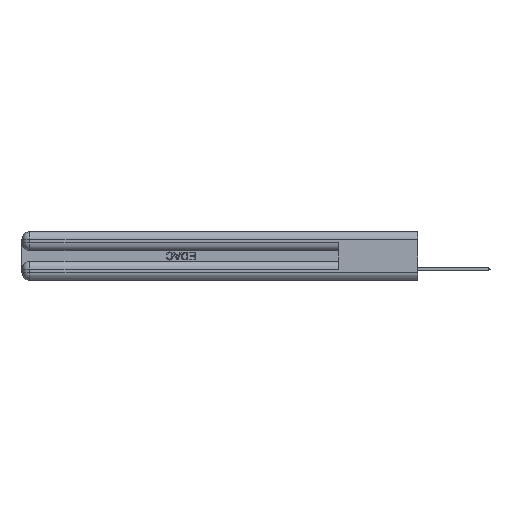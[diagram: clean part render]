
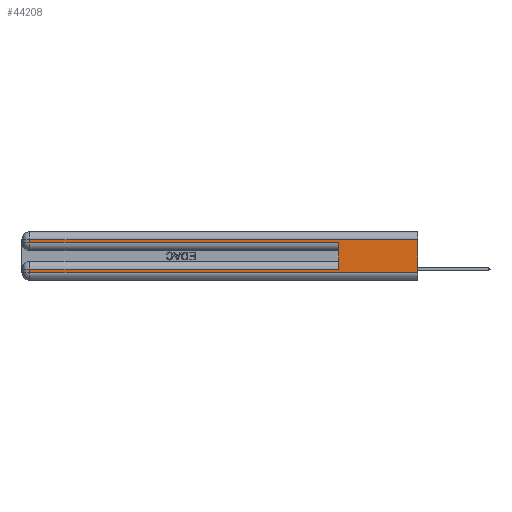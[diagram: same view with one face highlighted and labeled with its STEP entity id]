
A CAD part, left-side view. The second image highlights one B-rep face of the part: STEP entity #44208.
In plain terms, the highlighted planar face has unit normal (-1, 0, 0).
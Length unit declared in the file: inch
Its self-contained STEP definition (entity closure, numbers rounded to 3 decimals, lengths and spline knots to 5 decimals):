
#1173 = CARTESIAN_POINT ( 'NONE',  ( 0., 0.6, 0.085 ) ) ;
#1413 = VECTOR ( 'NONE', #7655, 39.37008 ) ;
#1732 = CARTESIAN_POINT ( 'NONE',  ( 0., 0., 0.06 ) ) ;
#3135 = LINE ( 'NONE', #49002, #53962 ) ;
#4906 = EDGE_CURVE ( 'NONE', #29374, #51223, #48851, .T. ) ;
#6257 = ORIENTED_EDGE ( 'NONE', *, *, #54126, .T. ) ;
#7452 = DIRECTION ( 'NONE',  ( 0., 0., -1. ) ) ;
#7655 = DIRECTION ( 'NONE',  ( 0., 0., -1. ) ) ;
#7700 = AXIS2_PLACEMENT_3D ( 'NONE', #39469, #31090, #48251 ) ;
#11592 = CARTESIAN_POINT ( 'NONE',  ( 0., 2.94, 0.085 ) ) ;
#13579 = EDGE_LOOP ( 'NONE', ( #37898, #44362, #16165, #43465, #49946, #6257, #46958, #41681 ) ) ;
#14281 = VECTOR ( 'NONE', #29861, 39.37008 ) ;
#14753 = VECTOR ( 'NONE', #7452, 39.37008 ) ;
#15265 = DIRECTION ( 'NONE',  ( 0., 0., 1. ) ) ;
#15511 = LINE ( 'NONE', #50221, #14753 ) ;
#15615 = LINE ( 'NONE', #54006, #1413 ) ;
#16165 = ORIENTED_EDGE ( 'NONE', *, *, #4906, .T. ) ;
#16483 = CARTESIAN_POINT ( 'NONE',  ( 0., 0., 0.085 ) ) ;
#16819 = VERTEX_POINT ( 'NONE', #1732 ) ;
#17747 = VECTOR ( 'NONE', #47881, 39.37008 ) ;
#18144 = EDGE_CURVE ( 'NONE', #26428, #54374, #3135, .T. ) ;
#19138 = EDGE_CURVE ( 'NONE', #21857, #16819, #35734, .T. ) ;
#19789 = DIRECTION ( 'NONE',  ( 0., 0., -1. ) ) ;
#21857 = VERTEX_POINT ( 'NONE', #54614 ) ;
#22884 = CARTESIAN_POINT ( 'NONE',  ( 0., 0.6, 0.285 ) ) ;
#23895 = CARTESIAN_POINT ( 'NONE',  ( 0., 0., 0.31 ) ) ;
#25116 = FACE_OUTER_BOUND ( 'NONE', #13579, .T. ) ;
#25306 = VERTEX_POINT ( 'NONE', #36333 ) ;
#26334 = VECTOR ( 'NONE', #53956, 39.37008 ) ;
#26428 = VERTEX_POINT ( 'NONE', #1173 ) ;
#27379 = PLANE ( 'NONE',  #7700 ) ;
#29374 = VERTEX_POINT ( 'NONE', #31067 ) ;
#29861 = DIRECTION ( 'NONE',  ( 0., 1., 0. ) ) ;
#31041 = EDGE_CURVE ( 'NONE', #25306, #29374, #33090, .T. ) ;
#31067 = CARTESIAN_POINT ( 'NONE',  ( 0., 2.94, 0.31 ) ) ;
#31090 = DIRECTION ( 'NONE',  ( 1., 0., 0. ) ) ;
#32414 = LINE ( 'NONE', #16483, #14281 ) ;
#33090 = LINE ( 'NONE', #23895, #26334 ) ;
#34194 = EDGE_CURVE ( 'NONE', #51223, #54374, #38763, .T. ) ;
#35734 = LINE ( 'NONE', #46307, #17747 ) ;
#36333 = CARTESIAN_POINT ( 'NONE',  ( 0., 0., 0.31 ) ) ;
#36867 = CARTESIAN_POINT ( 'NONE',  ( 0., 0., 0.285 ) ) ;
#37898 = ORIENTED_EDGE ( 'NONE', *, *, #50946, .F. ) ;
#38763 = LINE ( 'NONE', #36867, #41493 ) ;
#39469 = CARTESIAN_POINT ( 'NONE',  ( 0., 0., 0.37 ) ) ;
#41493 = VECTOR ( 'NONE', #54060, 39.37008 ) ;
#41681 = ORIENTED_EDGE ( 'NONE', *, *, #19138, .T. ) ;
#43465 = ORIENTED_EDGE ( 'NONE', *, *, #34194, .T. ) ;
#43824 = CARTESIAN_POINT ( 'NONE',  ( 0., 2.94, 0.285 ) ) ;
#43859 = VERTEX_POINT ( 'NONE', #11592 ) ;
#44208 = ADVANCED_FACE ( 'NONE', ( #25116 ), #27379, .F. ) ;
#44362 = ORIENTED_EDGE ( 'NONE', *, *, #31041, .T. ) ;
#46307 = CARTESIAN_POINT ( 'NONE',  ( 0., 0., 0.06 ) ) ;
#46958 = ORIENTED_EDGE ( 'NONE', *, *, #49742, .T. ) ;
#47881 = DIRECTION ( 'NONE',  ( 0., -1., 0. ) ) ;
#48251 = DIRECTION ( 'NONE',  ( 0., 0., -1. ) ) ;
#48851 = LINE ( 'NONE', #49561, #52203 ) ;
#49002 = CARTESIAN_POINT ( 'NONE',  ( 0., 0.6, 0.145 ) ) ;
#49561 = CARTESIAN_POINT ( 'NONE',  ( 0., 2.94, 0.37 ) ) ;
#49742 = EDGE_CURVE ( 'NONE', #43859, #21857, #15615, .T. ) ;
#49946 = ORIENTED_EDGE ( 'NONE', *, *, #18144, .F. ) ;
#50221 = CARTESIAN_POINT ( 'NONE',  ( 0., 0., 0.37 ) ) ;
#50946 = EDGE_CURVE ( 'NONE', #25306, #16819, #15511, .T. ) ;
#51223 = VERTEX_POINT ( 'NONE', #43824 ) ;
#52203 = VECTOR ( 'NONE', #19789, 39.37008 ) ;
#53956 = DIRECTION ( 'NONE',  ( 0., 1., 0. ) ) ;
#53962 = VECTOR ( 'NONE', #15265, 39.37008 ) ;
#54006 = CARTESIAN_POINT ( 'NONE',  ( 0., 2.94, 0.37 ) ) ;
#54060 = DIRECTION ( 'NONE',  ( 0., -1., 0. ) ) ;
#54126 = EDGE_CURVE ( 'NONE', #26428, #43859, #32414, .T. ) ;
#54374 = VERTEX_POINT ( 'NONE', #22884 ) ;
#54614 = CARTESIAN_POINT ( 'NONE',  ( 0., 2.94, 0.06 ) ) ;
